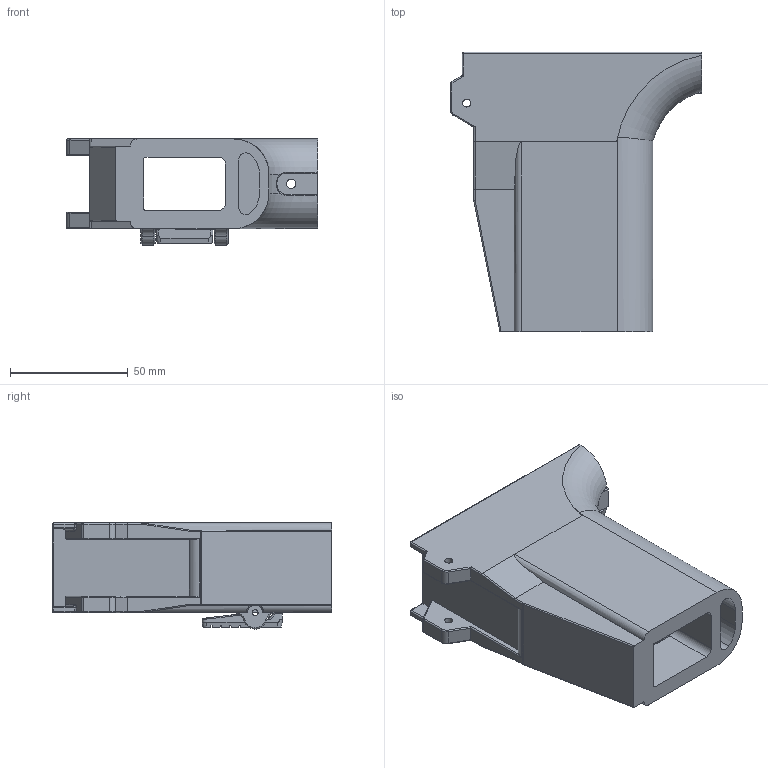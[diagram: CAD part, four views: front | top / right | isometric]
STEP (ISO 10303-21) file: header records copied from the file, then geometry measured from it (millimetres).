
FILE_DESCRIPTION(/* description */ (''),/* implementation_level */ '2;1');
FILE_NAME(/* name */ 'UZI Magwell.stp',/* time_stamp */ '2020-10-20T12:01:35+03:00',/* author */ (''),/* organization */ (''),/* preprocessor_version */ 'ST-DEVELOPER v15.2',/* originating_system */ 'Autodesk Translator Framework v2.0.0.5431',/* authorisation */ '');
FILE_SCHEMA (('AUTOMOTIVE_DESIGN { 1 0 10303 214 3 1 1 }'));
Length unit declared in the file: centimetre
Products named in the file (1): MOD9 UZI MAGWELL
Bounding box: 106.51 x 118.45 x 44.98 mm (x, y, z)
Volume: 217949.5 mm3; surface area: 53566.7 mm2
Topology: 2 solids, 2 shells, 642 faces, 1566 edges, 934 vertices
Faces by surface type: plane 330, cylinder 176, bspline 44, torus 39, cone 31, sphere 22
Full cylindrical faces by diameter (mm): 2.5 x2, 3.4 x2, 3.5 x2, 4 x2
Entity records: 19602 total; most frequent: CARTESIAN_POINT 4625, DIRECTION 3128, ORIENTED_EDGE 3094, EDGE_CURVE 1547, AXIS2_PLACEMENT_3D 1070, LINE 988, VECTOR 988, VERTEX_POINT 934
